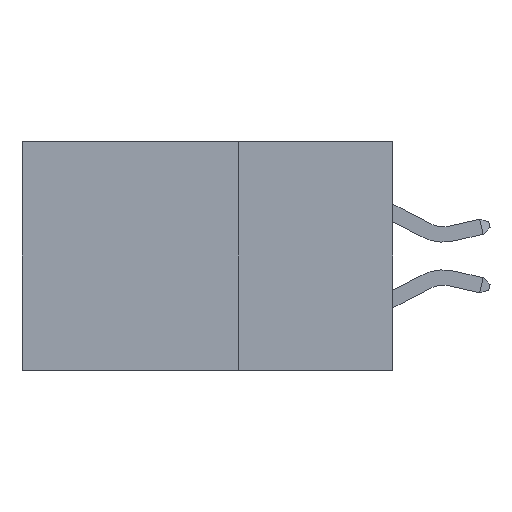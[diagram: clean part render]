
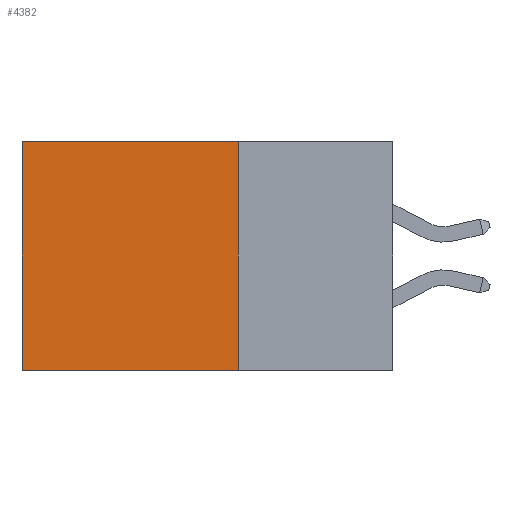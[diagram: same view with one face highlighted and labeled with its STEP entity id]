
A CAD part, left-side view. The second image highlights one B-rep face of the part: STEP entity #4382.
In plain terms, the highlighted planar face has unit normal (-1, 0, 0).
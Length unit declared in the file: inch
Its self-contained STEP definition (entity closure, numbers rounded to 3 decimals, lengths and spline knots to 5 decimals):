
#719 = DIRECTION ( 'NONE',  ( 0., 0., -1. ) ) ;
#1155 = PLANE ( 'NONE',  #26288 ) ;
#1547 = EDGE_CURVE ( 'NONE', #12347, #14936, #16133, .T. ) ;
#2141 = DIRECTION ( 'NONE',  ( 0., 1., 0. ) ) ;
#2626 = CARTESIAN_POINT ( 'NONE',  ( 0.2875, 0.6, 0. ) ) ;
#4382 = ADVANCED_FACE ( 'NONE', ( #21040 ), #1155, .F. ) ;
#5028 = DIRECTION ( 'NONE',  ( 0., 1., 0. ) ) ;
#6297 = LINE ( 'NONE', #25101, #17861 ) ;
#9671 = EDGE_CURVE ( 'NONE', #12347, #15973, #6297, .T. ) ;
#10225 = DIRECTION ( 'NONE',  ( 0., 0., -1. ) ) ;
#10868 = CARTESIAN_POINT ( 'NONE',  ( 0.2875, 0.25, 0. ) ) ;
#12347 = VERTEX_POINT ( 'NONE', #18511 ) ;
#12425 = CARTESIAN_POINT ( 'NONE',  ( 0.2875, 0.25, -0.37 ) ) ;
#13724 = VECTOR ( 'NONE', #5028, 39.37008 ) ;
#14237 = CARTESIAN_POINT ( 'NONE',  ( 0.2875, 0.6, -0.37 ) ) ;
#14744 = EDGE_LOOP ( 'NONE', ( #32948, #25926, #19847, #32437 ) ) ;
#14936 = VERTEX_POINT ( 'NONE', #18475 ) ;
#15973 = VERTEX_POINT ( 'NONE', #24360 ) ;
#16133 = LINE ( 'NONE', #25360, #13724 ) ;
#16848 = EDGE_CURVE ( 'NONE', #15973, #19860, #28273, .T. ) ;
#17861 = VECTOR ( 'NONE', #30229, 39.37008 ) ;
#18475 = CARTESIAN_POINT ( 'NONE',  ( 0.2875, 0.6, 0. ) ) ;
#18511 = CARTESIAN_POINT ( 'NONE',  ( 0.2875, 0.25, 0. ) ) ;
#19847 = ORIENTED_EDGE ( 'NONE', *, *, #9671, .F. ) ;
#19860 = VERTEX_POINT ( 'NONE', #14237 ) ;
#21040 = FACE_OUTER_BOUND ( 'NONE', #14744, .T. ) ;
#21147 = LINE ( 'NONE', #2626, #24383 ) ;
#21237 = DIRECTION ( 'NONE',  ( 1., 0., 0. ) ) ;
#21782 = EDGE_CURVE ( 'NONE', #14936, #19860, #21147, .T. ) ;
#23504 = VECTOR ( 'NONE', #2141, 39.37008 ) ;
#24360 = CARTESIAN_POINT ( 'NONE',  ( 0.2875, 0.25, -0.37 ) ) ;
#24383 = VECTOR ( 'NONE', #10225, 39.37008 ) ;
#25101 = CARTESIAN_POINT ( 'NONE',  ( 0.2875, 0.25, 0. ) ) ;
#25360 = CARTESIAN_POINT ( 'NONE',  ( 0.2875, 0.25, 0. ) ) ;
#25926 = ORIENTED_EDGE ( 'NONE', *, *, #16848, .F. ) ;
#26288 = AXIS2_PLACEMENT_3D ( 'NONE', #10868, #21237, #719 ) ;
#28273 = LINE ( 'NONE', #12425, #23504 ) ;
#30229 = DIRECTION ( 'NONE',  ( 0., 0., -1. ) ) ;
#32437 = ORIENTED_EDGE ( 'NONE', *, *, #1547, .T. ) ;
#32948 = ORIENTED_EDGE ( 'NONE', *, *, #21782, .T. ) ;
